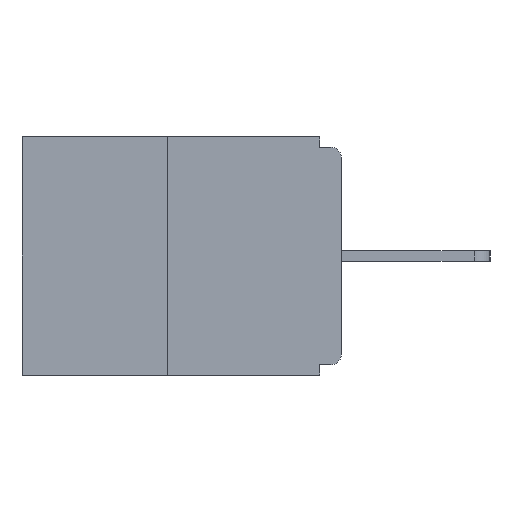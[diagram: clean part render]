
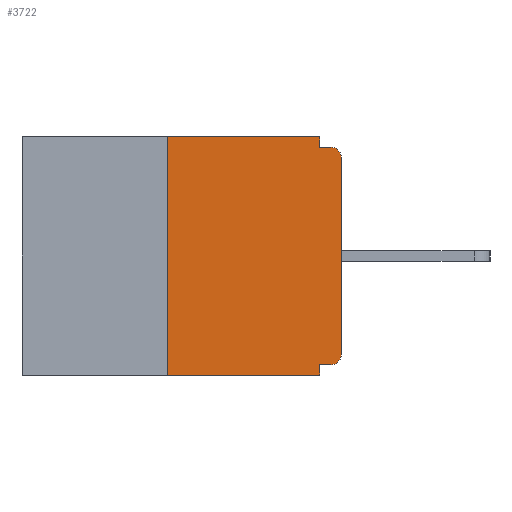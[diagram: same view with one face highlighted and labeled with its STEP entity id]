
A CAD part, left-side view. The second image highlights one B-rep face of the part: STEP entity #3722.
In plain terms, the highlighted planar face has unit normal (-1, 0, 0).
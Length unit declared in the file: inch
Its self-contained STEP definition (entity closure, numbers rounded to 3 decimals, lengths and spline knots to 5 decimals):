
#337 = VERTEX_POINT ( 'NONE', #8738 ) ;
#359 = DIRECTION ( 'NONE',  ( -1., 0., 0. ) ) ;
#501 = ORIENTED_EDGE ( 'NONE', *, *, #11704, .F. ) ;
#690 = CARTESIAN_POINT ( 'NONE',  ( 0., 0.25, 0. ) ) ;
#906 = CIRCLE ( 'NONE', #1347, 0.015 ) ;
#1029 = DIRECTION ( 'NONE',  ( 0., 0., -1. ) ) ;
#1248 = VERTEX_POINT ( 'NONE', #11914 ) ;
#1347 = AXIS2_PLACEMENT_3D ( 'NONE', #7753, #359, #2560 ) ;
#1375 = DIRECTION ( 'NONE',  ( 0., 1., 0. ) ) ;
#1410 = CARTESIAN_POINT ( 'NONE',  ( 0., 0.46, -0.343 ) ) ;
#1527 = LINE ( 'NONE', #12178, #1767 ) ;
#1647 = CARTESIAN_POINT ( 'NONE',  ( 0., 0.015, -0.313 ) ) ;
#1662 = ORIENTED_EDGE ( 'NONE', *, *, #9737, .F. ) ;
#1767 = VECTOR ( 'NONE', #5889, 39.37008 ) ;
#1826 = CARTESIAN_POINT ( 'NONE',  ( 0., 0., -0.03 ) ) ;
#2560 = DIRECTION ( 'NONE',  ( 0., 0., -1. ) ) ;
#2640 = EDGE_CURVE ( 'NONE', #8674, #11644, #10027, .T. ) ;
#2728 = VECTOR ( 'NONE', #1029, 39.37008 ) ;
#2780 = LINE ( 'NONE', #3749, #6277 ) ;
#2895 = ORIENTED_EDGE ( 'NONE', *, *, #5284, .T. ) ;
#3024 = CARTESIAN_POINT ( 'NONE',  ( 0., 0., 0. ) ) ;
#3122 = DIRECTION ( 'NONE',  ( 0., 0., -1. ) ) ;
#3175 = VERTEX_POINT ( 'NONE', #3841 ) ;
#3615 = VECTOR ( 'NONE', #8990, 39.37008 ) ;
#3722 = ADVANCED_FACE ( 'NONE', ( #8651 ), #12646, .F. ) ;
#3749 = CARTESIAN_POINT ( 'NONE',  ( 0., 0.031, 0. ) ) ;
#3795 = AXIS2_PLACEMENT_3D ( 'NONE', #8456, #8587, #3122 ) ;
#3841 = CARTESIAN_POINT ( 'NONE',  ( 0., 0.25, 0. ) ) ;
#3874 = EDGE_CURVE ( 'NONE', #8950, #9860, #906, .T. ) ;
#3929 = DIRECTION ( 'NONE',  ( -1., 0., 0. ) ) ;
#4005 = ORIENTED_EDGE ( 'NONE', *, *, #9267, .F. ) ;
#4388 = CIRCLE ( 'NONE', #11340, 0.015 ) ;
#4451 = LINE ( 'NONE', #5448, #6028 ) ;
#4952 = CARTESIAN_POINT ( 'NONE',  ( 0., 0., -0.015 ) ) ;
#5073 = VERTEX_POINT ( 'NONE', #12083 ) ;
#5284 = EDGE_CURVE ( 'NONE', #1248, #7869, #4388, .T. ) ;
#5448 = CARTESIAN_POINT ( 'NONE',  ( 0., 0., -0.328 ) ) ;
#5692 = ORIENTED_EDGE ( 'NONE', *, *, #5822, .T. ) ;
#5822 = EDGE_CURVE ( 'NONE', #7869, #8950, #12618, .T. ) ;
#5889 = DIRECTION ( 'NONE',  ( 0., -1., 0. ) ) ;
#5937 = DIRECTION ( 'NONE',  ( 0., -1., 0. ) ) ;
#6028 = VECTOR ( 'NONE', #1375, 39.37008 ) ;
#6277 = VECTOR ( 'NONE', #11050, 39.37008 ) ;
#6353 = CARTESIAN_POINT ( 'NONE',  ( 0., 0.031, -0.015 ) ) ;
#6596 = ORIENTED_EDGE ( 'NONE', *, *, #13097, .F. ) ;
#6728 = ORIENTED_EDGE ( 'NONE', *, *, #2640, .T. ) ;
#6902 = ORIENTED_EDGE ( 'NONE', *, *, #3874, .T. ) ;
#6997 = VERTEX_POINT ( 'NONE', #6353 ) ;
#7154 = DIRECTION ( 'NONE',  ( 0., 0., 1. ) ) ;
#7621 = VECTOR ( 'NONE', #7154, 39.37008 ) ;
#7753 = CARTESIAN_POINT ( 'NONE',  ( 0., 0.015, -0.03 ) ) ;
#7869 = VERTEX_POINT ( 'NONE', #8285 ) ;
#8233 = DIRECTION ( 'NONE',  ( 0., 0., -1. ) ) ;
#8285 = CARTESIAN_POINT ( 'NONE',  ( 0., 0., -0.313 ) ) ;
#8456 = CARTESIAN_POINT ( 'NONE',  ( 0., 0.46, 0. ) ) ;
#8587 = DIRECTION ( 'NONE',  ( 1., 0., 0. ) ) ;
#8651 = FACE_OUTER_BOUND ( 'NONE', #12171, .T. ) ;
#8674 = VERTEX_POINT ( 'NONE', #9626 ) ;
#8738 = CARTESIAN_POINT ( 'NONE',  ( 0., 0.031, -0.328 ) ) ;
#8950 = VERTEX_POINT ( 'NONE', #1826 ) ;
#8990 = DIRECTION ( 'NONE',  ( 0., -1., 0. ) ) ;
#9267 = EDGE_CURVE ( 'NONE', #3175, #5073, #1527, .T. ) ;
#9453 = CARTESIAN_POINT ( 'NONE',  ( 0., 0.031, -0.343 ) ) ;
#9626 = CARTESIAN_POINT ( 'NONE',  ( 0., 0.25, -0.343 ) ) ;
#9731 = DIRECTION ( 'NONE',  ( 0., 0., 1. ) ) ;
#9737 = EDGE_CURVE ( 'NONE', #5073, #6997, #2780, .T. ) ;
#9810 = EDGE_CURVE ( 'NONE', #6997, #9860, #11257, .T. ) ;
#9860 = VERTEX_POINT ( 'NONE', #13493 ) ;
#10027 = LINE ( 'NONE', #1410, #3615 ) ;
#10291 = VECTOR ( 'NONE', #5937, 39.37008 ) ;
#10681 = EDGE_CURVE ( 'NONE', #1248, #337, #4451, .T. ) ;
#11001 = CARTESIAN_POINT ( 'NONE',  ( 0., 0.031, -0.343 ) ) ;
#11050 = DIRECTION ( 'NONE',  ( 0., 0., -1. ) ) ;
#11191 = ORIENTED_EDGE ( 'NONE', *, *, #10681, .F. ) ;
#11257 = LINE ( 'NONE', #4952, #10291 ) ;
#11340 = AXIS2_PLACEMENT_3D ( 'NONE', #1647, #3929, #8233 ) ;
#11408 = LINE ( 'NONE', #690, #7621 ) ;
#11644 = VERTEX_POINT ( 'NONE', #11001 ) ;
#11693 = LINE ( 'NONE', #9453, #2728 ) ;
#11704 = EDGE_CURVE ( 'NONE', #8674, #3175, #11408, .T. ) ;
#11914 = CARTESIAN_POINT ( 'NONE',  ( 0., 0.015, -0.328 ) ) ;
#12014 = VECTOR ( 'NONE', #9731, 39.37008 ) ;
#12083 = CARTESIAN_POINT ( 'NONE',  ( 0., 0.031, 0. ) ) ;
#12171 = EDGE_LOOP ( 'NONE', ( #4005, #501, #6728, #6596, #11191, #2895, #5692, #6902, #12213, #1662 ) ) ;
#12178 = CARTESIAN_POINT ( 'NONE',  ( 0., 0.46, 0. ) ) ;
#12213 = ORIENTED_EDGE ( 'NONE', *, *, #9810, .F. ) ;
#12618 = LINE ( 'NONE', #3024, #12014 ) ;
#12646 = PLANE ( 'NONE',  #3795 ) ;
#13097 = EDGE_CURVE ( 'NONE', #337, #11644, #11693, .T. ) ;
#13493 = CARTESIAN_POINT ( 'NONE',  ( 0., 0.015, -0.015 ) ) ;
